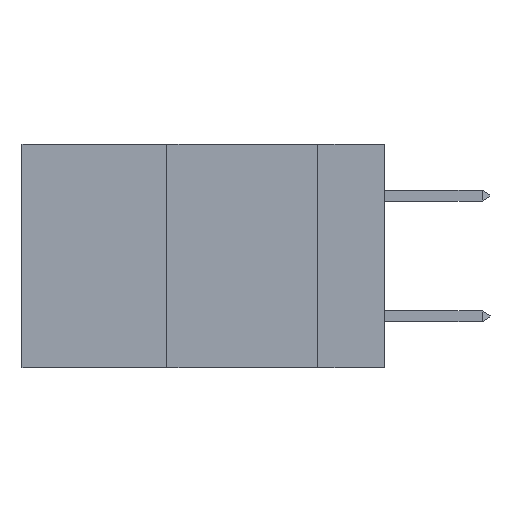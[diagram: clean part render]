
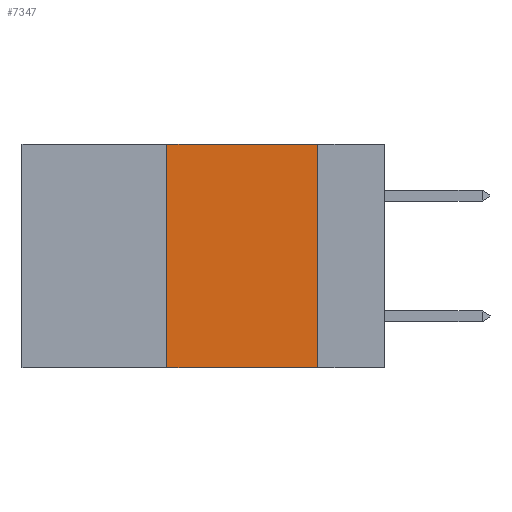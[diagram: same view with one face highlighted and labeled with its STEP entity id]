
A CAD part, left-side view. The second image highlights one B-rep face of the part: STEP entity #7347.
In plain terms, the highlighted planar face has unit normal (-1, 0, 0).
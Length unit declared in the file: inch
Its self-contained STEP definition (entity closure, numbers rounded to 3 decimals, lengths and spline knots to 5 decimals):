
#188 = DIRECTION ( 'NONE',  ( 0., 0., -1. ) ) ;
#1352 = VECTOR ( 'NONE', #5763, 39.37008 ) ;
#1377 = DIRECTION ( 'NONE',  ( 0., 0., 1. ) ) ;
#3731 = LINE ( 'NONE', #25244, #1352 ) ;
#4922 = CARTESIAN_POINT ( 'NONE',  ( 0., 0.6, 0. ) ) ;
#5259 = VECTOR ( 'NONE', #23062, 39.37008 ) ;
#5763 = DIRECTION ( 'NONE',  ( 0., 0., -1. ) ) ;
#6236 = CARTESIAN_POINT ( 'NONE',  ( 0., 0.36, -0.37 ) ) ;
#7279 = FACE_OUTER_BOUND ( 'NONE', #23619, .T. ) ;
#7347 = ADVANCED_FACE ( 'NONE', ( #7279 ), #16869, .F. ) ;
#8952 = LINE ( 'NONE', #16333, #14496 ) ;
#11561 = ORIENTED_EDGE ( 'NONE', *, *, #18514, .T. ) ;
#11730 = LINE ( 'NONE', #28538, #17026 ) ;
#12569 = EDGE_CURVE ( 'NONE', #19350, #21067, #3731, .T. ) ;
#12682 = CARTESIAN_POINT ( 'NONE',  ( 0., 0.11, -0.37 ) ) ;
#13474 = LINE ( 'NONE', #17877, #5259 ) ;
#13797 = VERTEX_POINT ( 'NONE', #6236 ) ;
#13991 = ORIENTED_EDGE ( 'NONE', *, *, #17951, .F. ) ;
#14128 = CARTESIAN_POINT ( 'NONE',  ( 0., 0.11, 0. ) ) ;
#14194 = AXIS2_PLACEMENT_3D ( 'NONE', #4922, #21729, #188 ) ;
#14496 = VECTOR ( 'NONE', #1377, 39.37008 ) ;
#16333 = CARTESIAN_POINT ( 'NONE',  ( 0., 0.36, 0. ) ) ;
#16869 = PLANE ( 'NONE',  #14194 ) ;
#17026 = VECTOR ( 'NONE', #21616, 39.37008 ) ;
#17698 = VERTEX_POINT ( 'NONE', #27156 ) ;
#17877 = CARTESIAN_POINT ( 'NONE',  ( 0., 0.6, 0. ) ) ;
#17951 = EDGE_CURVE ( 'NONE', #13797, #17698, #8952, .T. ) ;
#18514 = EDGE_CURVE ( 'NONE', #13797, #21067, #11730, .T. ) ;
#19350 = VERTEX_POINT ( 'NONE', #14128 ) ;
#19903 = ORIENTED_EDGE ( 'NONE', *, *, #24913, .F. ) ;
#20202 = ORIENTED_EDGE ( 'NONE', *, *, #12569, .F. ) ;
#21067 = VERTEX_POINT ( 'NONE', #12682 ) ;
#21616 = DIRECTION ( 'NONE',  ( 0., -1., 0. ) ) ;
#21729 = DIRECTION ( 'NONE',  ( 1., 0., 0. ) ) ;
#23062 = DIRECTION ( 'NONE',  ( 0., -1., 0. ) ) ;
#23619 = EDGE_LOOP ( 'NONE', ( #20202, #19903, #13991, #11561 ) ) ;
#24913 = EDGE_CURVE ( 'NONE', #17698, #19350, #13474, .T. ) ;
#25244 = CARTESIAN_POINT ( 'NONE',  ( 0., 0.11, 0. ) ) ;
#27156 = CARTESIAN_POINT ( 'NONE',  ( 0., 0.36, 0. ) ) ;
#28538 = CARTESIAN_POINT ( 'NONE',  ( 0., 0.6, -0.37 ) ) ;
